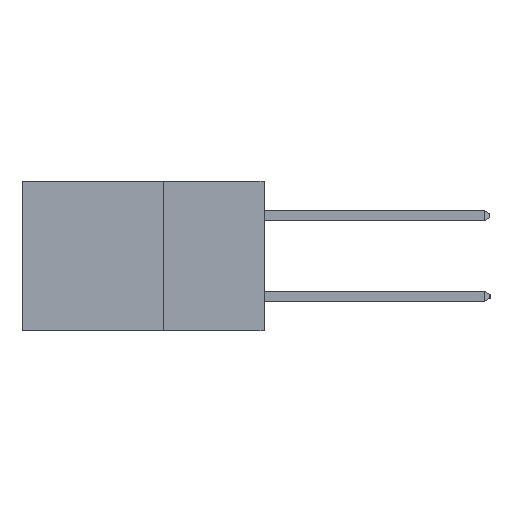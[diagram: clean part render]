
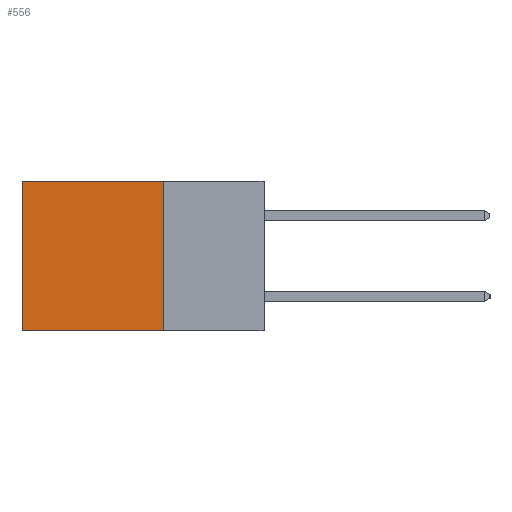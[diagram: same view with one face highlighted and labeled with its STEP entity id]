
A CAD part, left-side view. The second image highlights one B-rep face of the part: STEP entity #556.
In plain terms, the highlighted planar face has unit normal (-1, 0, 0).
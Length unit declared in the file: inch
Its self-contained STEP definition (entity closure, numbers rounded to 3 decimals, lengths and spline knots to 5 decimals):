
#556 = ADVANCED_FACE ( 'NONE', ( #11640 ), #8445, .F. ) ;
#686 = CARTESIAN_POINT ( 'NONE',  ( 0.2615, 0.25, 0. ) ) ;
#1079 = CARTESIAN_POINT ( 'NONE',  ( 0.2615, 0.6, 0. ) ) ;
#1265 = EDGE_CURVE ( 'NONE', #2287, #4891, #8644, .T. ) ;
#1944 = VECTOR ( 'NONE', #16565, 39.37008 ) ;
#2058 = AXIS2_PLACEMENT_3D ( 'NONE', #8462, #14709, #3260 ) ;
#2287 = VERTEX_POINT ( 'NONE', #8846 ) ;
#2545 = ORIENTED_EDGE ( 'NONE', *, *, #14452, .F. ) ;
#2670 = ORIENTED_EDGE ( 'NONE', *, *, #6091, .T. ) ;
#3260 = DIRECTION ( 'NONE',  ( 0., 0., -1. ) ) ;
#3715 = CARTESIAN_POINT ( 'NONE',  ( 0.2615, 0.25, 0. ) ) ;
#4218 = VECTOR ( 'NONE', #13601, 39.37008 ) ;
#4793 = VECTOR ( 'NONE', #10423, 39.37008 ) ;
#4891 = VERTEX_POINT ( 'NONE', #13423 ) ;
#5221 = LINE ( 'NONE', #3715, #4793 ) ;
#5712 = DIRECTION ( 'NONE',  ( 0., 0., -1. ) ) ;
#6091 = EDGE_CURVE ( 'NONE', #14669, #8744, #5221, .T. ) ;
#6899 = EDGE_LOOP ( 'NONE', ( #13784, #8869, #2545, #2670 ) ) ;
#8445 = PLANE ( 'NONE',  #2058 ) ;
#8462 = CARTESIAN_POINT ( 'NONE',  ( 0.2615, 0.25, -0.37 ) ) ;
#8467 = CARTESIAN_POINT ( 'NONE',  ( 0.2615, 0.6, -0.37 ) ) ;
#8644 = LINE ( 'NONE', #12233, #4218 ) ;
#8744 = VERTEX_POINT ( 'NONE', #1079 ) ;
#8846 = CARTESIAN_POINT ( 'NONE',  ( 0.2615, 0.25, -0.37 ) ) ;
#8869 = ORIENTED_EDGE ( 'NONE', *, *, #1265, .F. ) ;
#9603 = EDGE_CURVE ( 'NONE', #8744, #4891, #16702, .T. ) ;
#10423 = DIRECTION ( 'NONE',  ( 0., 1., 0. ) ) ;
#11640 = FACE_OUTER_BOUND ( 'NONE', #6899, .T. ) ;
#12233 = CARTESIAN_POINT ( 'NONE',  ( 0.2615, 0.25, -0.37 ) ) ;
#13199 = VECTOR ( 'NONE', #5712, 39.37008 ) ;
#13423 = CARTESIAN_POINT ( 'NONE',  ( 0.2615, 0.6, -0.37 ) ) ;
#13601 = DIRECTION ( 'NONE',  ( 0., 1., 0. ) ) ;
#13784 = ORIENTED_EDGE ( 'NONE', *, *, #9603, .T. ) ;
#14452 = EDGE_CURVE ( 'NONE', #14669, #2287, #16792, .T. ) ;
#14669 = VERTEX_POINT ( 'NONE', #686 ) ;
#14709 = DIRECTION ( 'NONE',  ( 1., 0., 0. ) ) ;
#15138 = CARTESIAN_POINT ( 'NONE',  ( 0.2615, 0.25, -0.37 ) ) ;
#16565 = DIRECTION ( 'NONE',  ( 0., 0., -1. ) ) ;
#16702 = LINE ( 'NONE', #8467, #1944 ) ;
#16792 = LINE ( 'NONE', #15138, #13199 ) ;
